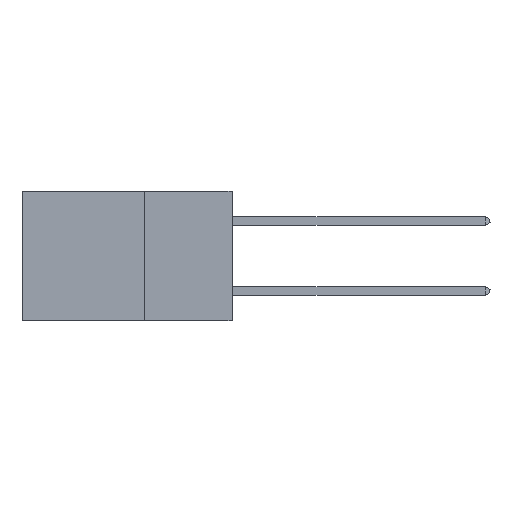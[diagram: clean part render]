
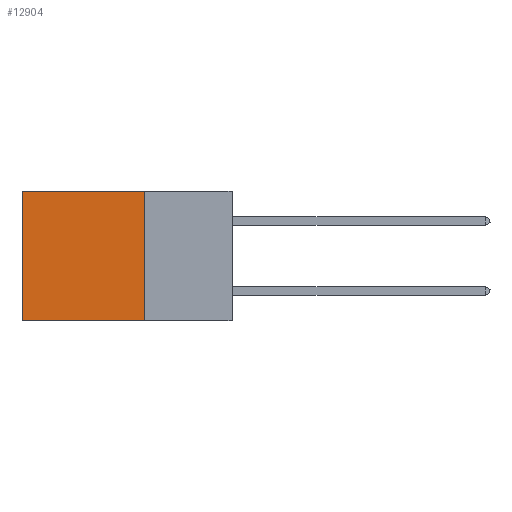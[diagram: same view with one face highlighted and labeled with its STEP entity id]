
A CAD part, left-side view. The second image highlights one B-rep face of the part: STEP entity #12904.
In plain terms, the highlighted planar face has unit normal (-1, 0, 0).
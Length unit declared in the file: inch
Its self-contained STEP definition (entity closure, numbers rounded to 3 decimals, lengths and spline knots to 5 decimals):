
#3 = EDGE_CURVE ( 'NONE', #14039, #10401, #11305, .T. ) ;
#782 = CARTESIAN_POINT ( 'NONE',  ( 0.2875, 0.25, 0. ) ) ;
#1381 = CARTESIAN_POINT ( 'NONE',  ( 0.2875, 0.6, -0.37 ) ) ;
#1618 = DIRECTION ( 'NONE',  ( 1., 0., 0. ) ) ;
#1682 = ORIENTED_EDGE ( 'NONE', *, *, #12951, .F. ) ;
#2174 = LINE ( 'NONE', #3880, #2607 ) ;
#2607 = VECTOR ( 'NONE', #12642, 39.37008 ) ;
#2849 = DIRECTION ( 'NONE',  ( 0., 1., 0. ) ) ;
#3880 = CARTESIAN_POINT ( 'NONE',  ( 0.2875, 0.25, 0. ) ) ;
#4069 = CARTESIAN_POINT ( 'NONE',  ( 0.2875, 0.6, 0. ) ) ;
#4193 = DIRECTION ( 'NONE',  ( 0., 0., -1. ) ) ;
#5119 = EDGE_LOOP ( 'NONE', ( #7049, #9987, #1682, #5844 ) ) ;
#5844 = ORIENTED_EDGE ( 'NONE', *, *, #11603, .T. ) ;
#6832 = CARTESIAN_POINT ( 'NONE',  ( 0.2875, 0.25, 0. ) ) ;
#7049 = ORIENTED_EDGE ( 'NONE', *, *, #3, .T. ) ;
#8006 = VECTOR ( 'NONE', #4193, 39.37008 ) ;
#8612 = AXIS2_PLACEMENT_3D ( 'NONE', #6832, #1618, #10658 ) ;
#9285 = CARTESIAN_POINT ( 'NONE',  ( 0.2875, 0.25, -0.37 ) ) ;
#9404 = PLANE ( 'NONE',  #8612 ) ;
#9987 = ORIENTED_EDGE ( 'NONE', *, *, #13378, .F. ) ;
#10401 = VERTEX_POINT ( 'NONE', #1381 ) ;
#10658 = DIRECTION ( 'NONE',  ( 0., 0., -1. ) ) ;
#11071 = LINE ( 'NONE', #9285, #14838 ) ;
#11084 = LINE ( 'NONE', #14217, #14167 ) ;
#11305 = LINE ( 'NONE', #4069, #8006 ) ;
#11458 = VERTEX_POINT ( 'NONE', #782 ) ;
#11603 = EDGE_CURVE ( 'NONE', #11458, #14039, #2174, .T. ) ;
#12358 = CARTESIAN_POINT ( 'NONE',  ( 0.2875, 0.25, -0.37 ) ) ;
#12642 = DIRECTION ( 'NONE',  ( 0., 1., 0. ) ) ;
#12904 = ADVANCED_FACE ( 'NONE', ( #14849 ), #9404, .F. ) ;
#12951 = EDGE_CURVE ( 'NONE', #11458, #14913, #11084, .T. ) ;
#13378 = EDGE_CURVE ( 'NONE', #14913, #10401, #11071, .T. ) ;
#14039 = VERTEX_POINT ( 'NONE', #15180 ) ;
#14167 = VECTOR ( 'NONE', #15300, 39.37008 ) ;
#14217 = CARTESIAN_POINT ( 'NONE',  ( 0.2875, 0.25, 0. ) ) ;
#14838 = VECTOR ( 'NONE', #2849, 39.37008 ) ;
#14849 = FACE_OUTER_BOUND ( 'NONE', #5119, .T. ) ;
#14913 = VERTEX_POINT ( 'NONE', #12358 ) ;
#15180 = CARTESIAN_POINT ( 'NONE',  ( 0.2875, 0.6, 0. ) ) ;
#15300 = DIRECTION ( 'NONE',  ( 0., 0., -1. ) ) ;
